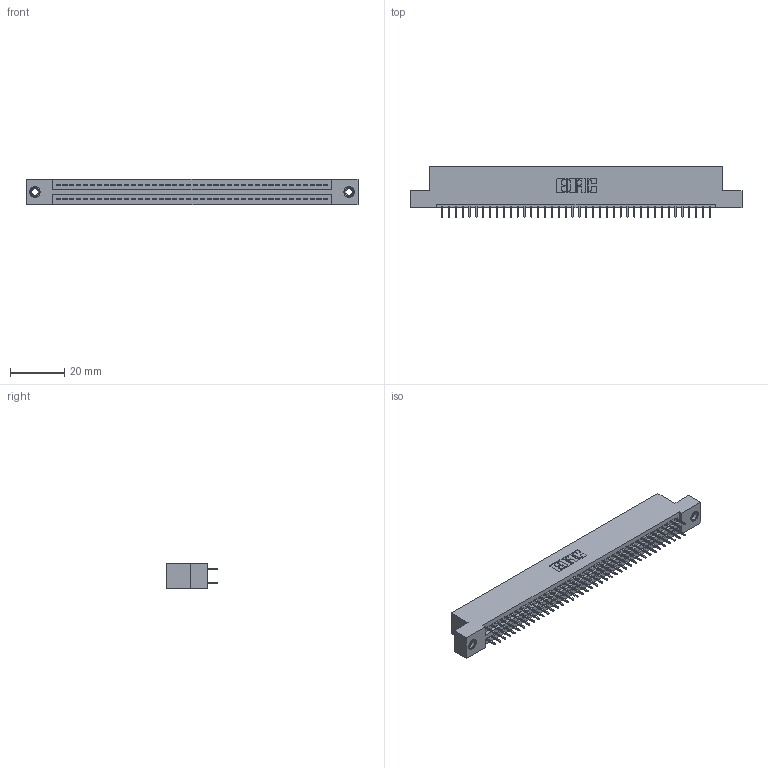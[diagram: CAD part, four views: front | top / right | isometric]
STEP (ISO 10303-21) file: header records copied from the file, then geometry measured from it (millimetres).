
FILE_DESCRIPTION (( 'STEP AP203' ), '1' );
FILE_NAME ('845-080-525-207.STEP', '2020-09-24T00:54:00', ( '' ), ( '' ), 'SwSTEP 2.0', 'SolidWorks 2020', '' );
FILE_SCHEMA (( 'CONFIG_CONTROL_DESIGN' ));
Length unit declared in the file: inch
Products named in the file (4): 345-250-001_345-250-005-103; 845 Part_Flush Mounting Lugs - 0.156 Dia-TI; 345-292-001_345-293-125; 845-080-525-207
Assembly tree (83 placements, depth 2):
  845-080-525-207
    845 Part_Flush Mounting Lugs - 0.156 Dia-TI
    345-292-001_345-293-125  x80
    345-250-001_345-250-005-103  x2
Bounding box: 122.81 x 18.72 x 9.4 mm (x, y, z)
Volume: 11766 mm3; surface area: 16984.5 mm2
Topology: 83 solids, 83 shells, 4506 faces, 12717 edges, 8150 vertices
Faces by surface type: plane 3232, cylinder 1258, cone 12, torus 4
Entity records: 32914 total; most frequent: CARTESIAN_POINT 5499, ORIENTED_EDGE 5426, DIRECTION 4879, EDGE_CURVE 2713, LINE 2405, VECTOR 2405, VERTEX_POINT 1800, AXIS2_PLACEMENT_3D 1237
